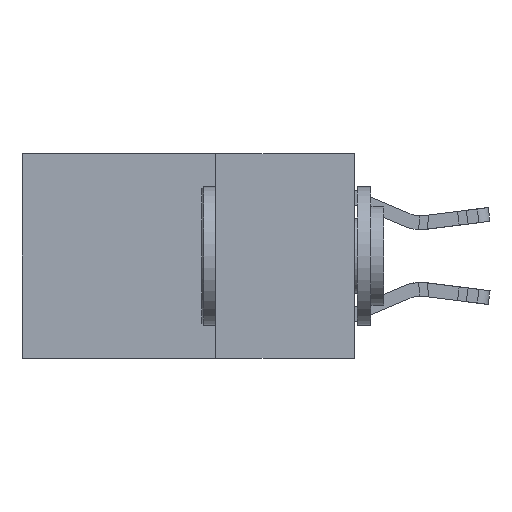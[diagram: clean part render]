
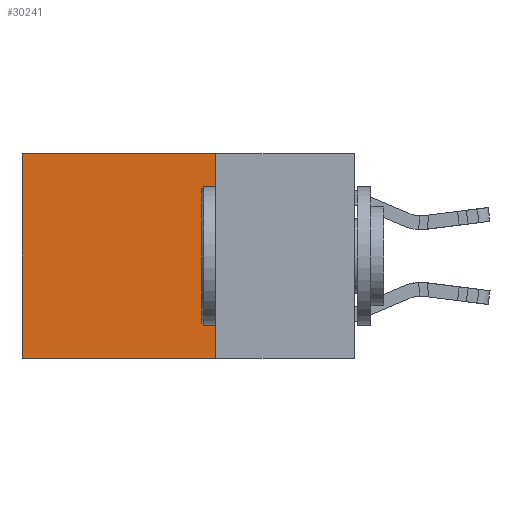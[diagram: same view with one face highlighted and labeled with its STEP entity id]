
A CAD part, left-side view. The second image highlights one B-rep face of the part: STEP entity #30241.
In plain terms, the highlighted planar face has unit normal (-1, 0, 0).
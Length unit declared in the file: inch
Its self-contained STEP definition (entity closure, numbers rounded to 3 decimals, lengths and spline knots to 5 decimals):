
#612 = EDGE_CURVE ( 'NONE', #22500, #10555, #27139, .T. ) ;
#1186 = LINE ( 'NONE', #20583, #26353 ) ;
#1240 = VECTOR ( 'NONE', #23823, 39.37008 ) ;
#3976 = FACE_OUTER_BOUND ( 'NONE', #8137, .T. ) ;
#4018 = VERTEX_POINT ( 'NONE', #7152 ) ;
#5991 = DIRECTION ( 'NONE',  ( 0., 1., 0. ) ) ;
#6107 = CARTESIAN_POINT ( 'NONE',  ( 0.2625, 0.6, 0. ) ) ;
#7152 = CARTESIAN_POINT ( 'NONE',  ( 0.2625, 0.6, -0.37 ) ) ;
#7392 = DIRECTION ( 'NONE',  ( 0., 0., -1. ) ) ;
#7885 = ORIENTED_EDGE ( 'NONE', *, *, #11705, .F. ) ;
#8137 = EDGE_LOOP ( 'NONE', ( #22563, #7885, #31180, #21641 ) ) ;
#8722 = AXIS2_PLACEMENT_3D ( 'NONE', #10297, #27304, #12744 ) ;
#8866 = VECTOR ( 'NONE', #7392, 39.37008 ) ;
#9052 = CARTESIAN_POINT ( 'NONE',  ( 0.2625, 0.6, 0. ) ) ;
#10151 = DIRECTION ( 'NONE',  ( 0., 1., 0. ) ) ;
#10297 = CARTESIAN_POINT ( 'NONE',  ( 0.2625, 0.25, 0. ) ) ;
#10555 = VERTEX_POINT ( 'NONE', #12851 ) ;
#11269 = CARTESIAN_POINT ( 'NONE',  ( 0.2625, 0.25, 0. ) ) ;
#11387 = EDGE_CURVE ( 'NONE', #24288, #4018, #16089, .T. ) ;
#11705 = EDGE_CURVE ( 'NONE', #10555, #4018, #1186, .T. ) ;
#12744 = DIRECTION ( 'NONE',  ( 0., 0., -1. ) ) ;
#12851 = CARTESIAN_POINT ( 'NONE',  ( 0.2625, 0.25, -0.37 ) ) ;
#16089 = LINE ( 'NONE', #6107, #8866 ) ;
#16679 = LINE ( 'NONE', #24704, #23128 ) ;
#19583 = EDGE_CURVE ( 'NONE', #22500, #24288, #16679, .T. ) ;
#20583 = CARTESIAN_POINT ( 'NONE',  ( 0.2625, 0.25, -0.37 ) ) ;
#21375 = CARTESIAN_POINT ( 'NONE',  ( 0.2625, 0.25, 0. ) ) ;
#21641 = ORIENTED_EDGE ( 'NONE', *, *, #19583, .T. ) ;
#22500 = VERTEX_POINT ( 'NONE', #11269 ) ;
#22563 = ORIENTED_EDGE ( 'NONE', *, *, #11387, .T. ) ;
#23128 = VECTOR ( 'NONE', #10151, 39.37008 ) ;
#23823 = DIRECTION ( 'NONE',  ( 0., 0., -1. ) ) ;
#24288 = VERTEX_POINT ( 'NONE', #9052 ) ;
#24704 = CARTESIAN_POINT ( 'NONE',  ( 0.2625, 0.25, 0. ) ) ;
#24875 = PLANE ( 'NONE',  #8722 ) ;
#26353 = VECTOR ( 'NONE', #5991, 39.37008 ) ;
#27139 = LINE ( 'NONE', #21375, #1240 ) ;
#27304 = DIRECTION ( 'NONE',  ( 1., 0., 0. ) ) ;
#30241 = ADVANCED_FACE ( 'NONE', ( #3976 ), #24875, .F. ) ;
#31180 = ORIENTED_EDGE ( 'NONE', *, *, #612, .F. ) ;
